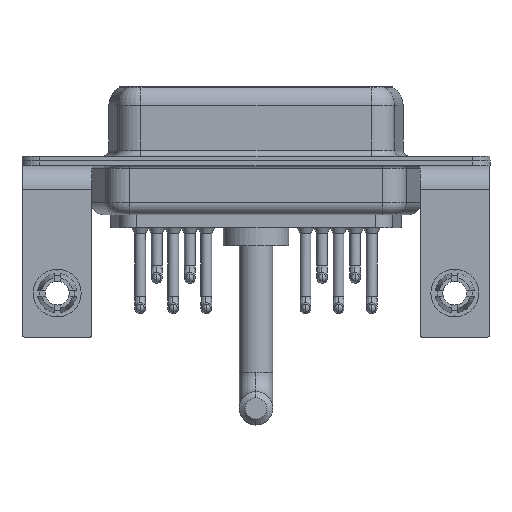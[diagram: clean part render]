
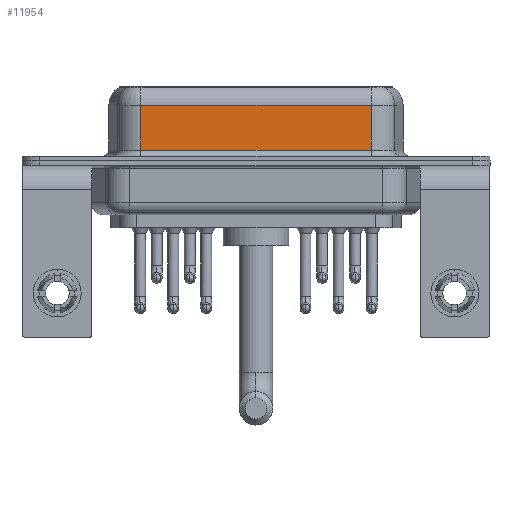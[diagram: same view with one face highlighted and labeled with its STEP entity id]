
A CAD part, front view. The second image highlights one B-rep face of the part: STEP entity #11954.
In plain terms, the highlighted planar face has unit normal (0, -1, 0).
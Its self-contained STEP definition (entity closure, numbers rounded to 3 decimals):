
#391 = VERTEX_POINT ( 'NONE', #12741 ) ;
#774 = CARTESIAN_POINT ( 'NONE',  ( 7.013, -3.95, 6.4 ) ) ;
#1180 = LINE ( 'NONE', #774, #11308 ) ;
#1474 = EDGE_CURVE ( 'NONE', #17869, #3070, #14609, .T. ) ;
#1528 = DIRECTION ( 'NONE',  ( -1., 0., 0. ) ) ;
#1799 = ORIENTED_EDGE ( 'NONE', *, *, #2301, .T. ) ;
#2301 = EDGE_CURVE ( 'NONE', #391, #3070, #10998, .T. ) ;
#2984 = DIRECTION ( 'NONE',  ( 0., 1., 0. ) ) ;
#3070 = VERTEX_POINT ( 'NONE', #18646 ) ;
#3097 = FACE_OUTER_BOUND ( 'NONE', #10567, .T. ) ;
#3463 = VECTOR ( 'NONE', #14311, 1000. ) ;
#4512 = VERTEX_POINT ( 'NONE', #10338 ) ;
#4806 = CARTESIAN_POINT ( 'NONE',  ( 26.287, -3.95, 6.4 ) ) ;
#5009 = CARTESIAN_POINT ( 'NONE',  ( 26.287, -3.95, 6.4 ) ) ;
#5773 = DIRECTION ( 'NONE',  ( 0., 0., -1. ) ) ;
#5817 = VECTOR ( 'NONE', #11500, 1000. ) ;
#7720 = EDGE_CURVE ( 'NONE', #17869, #4512, #19313, .T. ) ;
#9741 = ORIENTED_EDGE ( 'NONE', *, *, #1474, .F. ) ;
#10338 = CARTESIAN_POINT ( 'NONE',  ( 7.013, -3.95, 4.65 ) ) ;
#10567 = EDGE_LOOP ( 'NONE', ( #9741, #10755, #14493, #1799 ) ) ;
#10755 = ORIENTED_EDGE ( 'NONE', *, *, #7720, .T. ) ;
#10820 = VECTOR ( 'NONE', #1528, 1000. ) ;
#10998 = LINE ( 'NONE', #14116, #3463 ) ;
#11308 = VECTOR ( 'NONE', #5773, 1000. ) ;
#11500 = DIRECTION ( 'NONE',  ( 0., 0., -1. ) ) ;
#11954 = ADVANCED_FACE ( 'NONE', ( #3097 ), #17911, .F. ) ;
#12583 = EDGE_CURVE ( 'NONE', #4512, #391, #1180, .T. ) ;
#12741 = CARTESIAN_POINT ( 'NONE',  ( 7.013, -3.95, 0.9 ) ) ;
#14116 = CARTESIAN_POINT ( 'NONE',  ( 26.287, -3.95, 0.9 ) ) ;
#14311 = DIRECTION ( 'NONE',  ( 1., 0., 0. ) ) ;
#14493 = ORIENTED_EDGE ( 'NONE', *, *, #12583, .T. ) ;
#14609 = LINE ( 'NONE', #5009, #5817 ) ;
#14645 = CARTESIAN_POINT ( 'NONE',  ( 26.287, -3.95, 4.65 ) ) ;
#17388 = CARTESIAN_POINT ( 'NONE',  ( 26.287, -3.95, 4.65 ) ) ;
#17591 = DIRECTION ( 'NONE',  ( 0., 0., 1. ) ) ;
#17730 = AXIS2_PLACEMENT_3D ( 'NONE', #4806, #2984, #17591 ) ;
#17869 = VERTEX_POINT ( 'NONE', #17388 ) ;
#17911 = PLANE ( 'NONE',  #17730 ) ;
#18646 = CARTESIAN_POINT ( 'NONE',  ( 26.287, -3.95, 0.9 ) ) ;
#19313 = LINE ( 'NONE', #14645, #10820 ) ;
